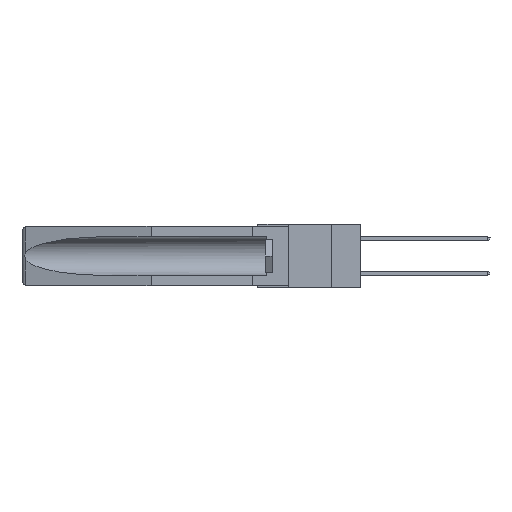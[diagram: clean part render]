
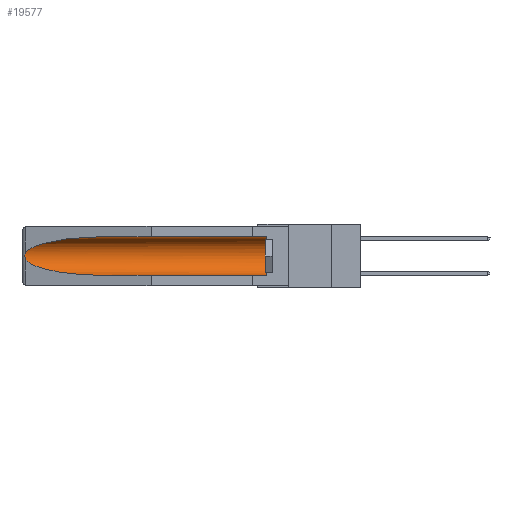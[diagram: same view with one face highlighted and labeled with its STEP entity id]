
A CAD part, left-side view. The second image highlights one B-rep face of the part: STEP entity #19577.
In plain terms, the highlighted cylindrical face has radius 2.857 mm (diameter 5.715 mm), a partial arc.
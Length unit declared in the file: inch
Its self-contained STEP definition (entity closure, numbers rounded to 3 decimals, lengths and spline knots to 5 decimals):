
#280 = ORIENTED_EDGE ( 'NONE', *, *, #12458, .T. ) ;
#439 = EDGE_LOOP ( 'NONE', ( #14274, #21212, #25123, #18052, #280, #16317 ) ) ;
#600 = CARTESIAN_POINT ( 'NONE',  ( 0.26537, 1.52718, -0.19328 ) ) ;
#751 = CARTESIAN_POINT ( 'NONE',  ( 0.155, 1.07973, -0.284 ) ) ;
#817 = FACE_OUTER_BOUND ( 'NONE', #439, .T. ) ;
#1694 = B_SPLINE_CURVE_WITH_KNOTS ( 'NONE', 3,
 ( #26901, #15311, #28922, #22227, #19767, #2136, #29195, #24710, #4008, #22319 ),
 .UNSPECIFIED., .F., .F.,
 ( 4, 2, 2, 2, 4 ),
 ( 0., 0.00029, 0.00058, 0.00087, 0.00117 ),
 .UNSPECIFIED. ) ;
#2136 = CARTESIAN_POINT ( 'NONE',  ( 0.2675, 1.53308, -0.17534 ) ) ;
#2812 = VERTEX_POINT ( 'NONE', #751 ) ;
#3489 =( BOUNDED_CURVE ( )  B_SPLINE_CURVE ( 3, ( #14317, #21427, #7489, #7878 ),
 .UNSPECIFIED., .F., .F. ) 
 B_SPLINE_CURVE_WITH_KNOTS ( ( 4, 4 ),
 ( 4.71239, 6.08839 ),
 .UNSPECIFIED. ) 
 CURVE ( )  GEOMETRIC_REPRESENTATION_ITEM ( )  RATIONAL_B_SPLINE_CURVE ( ( 1., 0.848, 0.848, 1. ) ) 
 REPRESENTATION_ITEM ( '' )  );
#3645 = VERTEX_POINT ( 'NONE', #8259 ) ;
#4008 = CARTESIAN_POINT ( 'NONE',  ( 0.26597, 1.5296, -0.19026 ) ) ;
#5066 = CARTESIAN_POINT ( 'NONE',  ( 0.155, -0.30754, -0.1715 ) ) ;
#5449 = CARTESIAN_POINT ( 'NONE',  ( 0.25451, 1.48313, -0.24835 ) ) ;
#7012 = VERTEX_POINT ( 'NONE', #25537 ) ;
#7094 = AXIS2_PLACEMENT_3D ( 'NONE', #5066, #16646, #27873 ) ;
#7489 = CARTESIAN_POINT ( 'NONE',  ( 0.25451, 1.48313, -0.09465 ) ) ;
#7878 = CARTESIAN_POINT ( 'NONE',  ( 0.26537, 1.52718, -0.14972 ) ) ;
#7989 = LINE ( 'NONE', #18436, #18620 ) ;
#8259 = CARTESIAN_POINT ( 'NONE',  ( 0.155, 1.07973, -0.059 ) ) ;
#8355 = VECTOR ( 'NONE', #18751, 39.37008 ) ;
#9532 = EDGE_CURVE ( 'NONE', #21864, #2812, #28587, .T. ) ;
#10244 = CIRCLE ( 'NONE', #25755, 0.1125 ) ;
#11250 = DIRECTION ( 'NONE',  ( 0., -1., 0. ) ) ;
#11327 = VERTEX_POINT ( 'NONE', #25188 ) ;
#12458 = EDGE_CURVE ( 'NONE', #28496, #7012, #10244, .T. ) ;
#12866 = CYLINDRICAL_SURFACE ( 'NONE', #7094, 0.1125 ) ;
#13532 = CARTESIAN_POINT ( 'NONE',  ( 0.155, 0.126, -0.1715 ) ) ;
#14274 = ORIENTED_EDGE ( 'NONE', *, *, #18038, .T. ) ;
#14317 = CARTESIAN_POINT ( 'NONE',  ( 0.155, 1.07973, -0.059 ) ) ;
#15311 = CARTESIAN_POINT ( 'NONE',  ( 0.26597, 1.52961, -0.15275 ) ) ;
#16317 = ORIENTED_EDGE ( 'NONE', *, *, #23481, .T. ) ;
#16443 = CARTESIAN_POINT ( 'NONE',  ( 0.155, 1.07973, -0.284 ) ) ;
#16646 = DIRECTION ( 'NONE',  ( 0., 1., 0. ) ) ;
#16783 = EDGE_CURVE ( 'NONE', #11327, #21864, #1694, .T. ) ;
#17231 = LINE ( 'NONE', #27401, #8355 ) ;
#18010 = DIRECTION ( 'NONE',  ( 0., 0., 1. ) ) ;
#18038 = EDGE_CURVE ( 'NONE', #3645, #11327, #3489, .T. ) ;
#18052 = ORIENTED_EDGE ( 'NONE', *, *, #23133, .F. ) ;
#18436 = CARTESIAN_POINT ( 'NONE',  ( 0.155, -0.30754, -0.059 ) ) ;
#18620 = VECTOR ( 'NONE', #27562, 39.37008 ) ;
#18751 = DIRECTION ( 'NONE',  ( 0., 1., 0. ) ) ;
#18797 = CARTESIAN_POINT ( 'NONE',  ( 0.155, 0.126, -0.284 ) ) ;
#19577 = ADVANCED_FACE ( 'NONE', ( #817 ), #12866, .F. ) ;
#19767 = CARTESIAN_POINT ( 'NONE',  ( 0.2675, 1.53308, -0.16763 ) ) ;
#21212 = ORIENTED_EDGE ( 'NONE', *, *, #16783, .T. ) ;
#21427 = CARTESIAN_POINT ( 'NONE',  ( 0.21114, 1.30732, -0.059 ) ) ;
#21864 = VERTEX_POINT ( 'NONE', #28294 ) ;
#22227 = CARTESIAN_POINT ( 'NONE',  ( 0.2673, 1.5327, -0.16383 ) ) ;
#22319 = CARTESIAN_POINT ( 'NONE',  ( 0.26537, 1.52718, -0.19328 ) ) ;
#23133 = EDGE_CURVE ( 'NONE', #28496, #2812, #17231, .T. ) ;
#23269 = CARTESIAN_POINT ( 'NONE',  ( 0.21114, 1.30732, -0.284 ) ) ;
#23481 = EDGE_CURVE ( 'NONE', #7012, #3645, #7989, .T. ) ;
#24710 = CARTESIAN_POINT ( 'NONE',  ( 0.26655, 1.53094, -0.18657 ) ) ;
#25123 = ORIENTED_EDGE ( 'NONE', *, *, #9532, .T. ) ;
#25188 = CARTESIAN_POINT ( 'NONE',  ( 0.26537, 1.52718, -0.14972 ) ) ;
#25537 = CARTESIAN_POINT ( 'NONE',  ( 0.155, 0.126, -0.059 ) ) ;
#25755 = AXIS2_PLACEMENT_3D ( 'NONE', #13532, #11250, #18010 ) ;
#26901 = CARTESIAN_POINT ( 'NONE',  ( 0.26537, 1.52718, -0.14972 ) ) ;
#27401 = CARTESIAN_POINT ( 'NONE',  ( 0.155, -0.30754, -0.284 ) ) ;
#27562 = DIRECTION ( 'NONE',  ( 0., 1., 0. ) ) ;
#27873 = DIRECTION ( 'NONE',  ( 0., 0., 1. ) ) ;
#28294 = CARTESIAN_POINT ( 'NONE',  ( 0.26537, 1.52718, -0.19328 ) ) ;
#28496 = VERTEX_POINT ( 'NONE', #18797 ) ;
#28587 =( BOUNDED_CURVE ( )  B_SPLINE_CURVE ( 3, ( #600, #5449, #23269, #16443 ),
 .UNSPECIFIED., .F., .F. ) 
 B_SPLINE_CURVE_WITH_KNOTS ( ( 4, 4 ),
 ( 0.1948, 1.5708 ),
 .UNSPECIFIED. ) 
 CURVE ( )  GEOMETRIC_REPRESENTATION_ITEM ( )  RATIONAL_B_SPLINE_CURVE ( ( 1., 0.848, 0.848, 1. ) ) 
 REPRESENTATION_ITEM ( '' )  );
#28922 = CARTESIAN_POINT ( 'NONE',  ( 0.26654, 1.53092, -0.15636 ) ) ;
#29195 = CARTESIAN_POINT ( 'NONE',  ( 0.2673, 1.53269, -0.17917 ) ) ;
